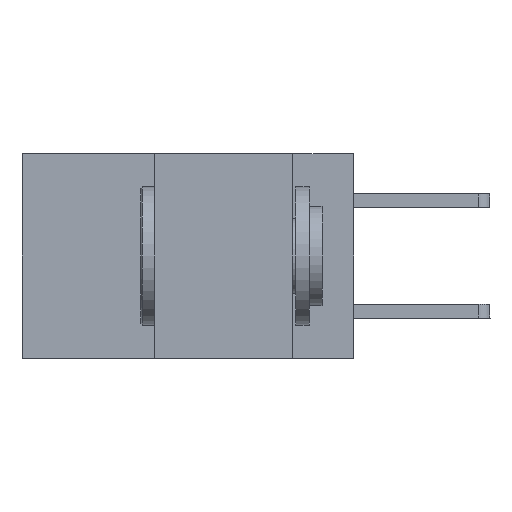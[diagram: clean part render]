
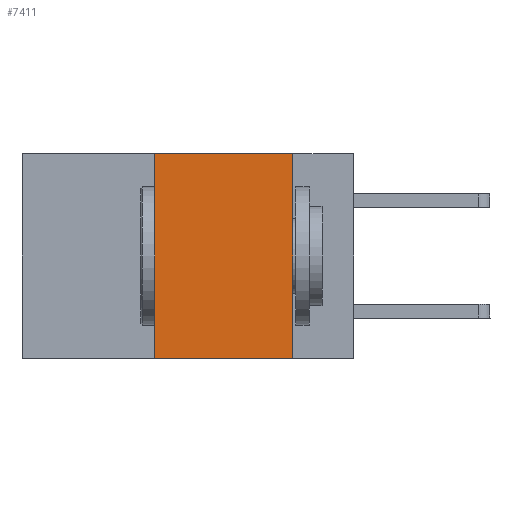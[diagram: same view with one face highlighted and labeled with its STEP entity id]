
A CAD part, left-side view. The second image highlights one B-rep face of the part: STEP entity #7411.
In plain terms, the highlighted planar face has unit normal (-1, 0, 0).
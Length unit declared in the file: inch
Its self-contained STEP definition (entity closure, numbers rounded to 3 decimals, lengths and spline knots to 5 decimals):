
#1052 = DIRECTION ( 'NONE',  ( 0., 0., -1. ) ) ;
#1598 = VERTEX_POINT ( 'NONE', #10853 ) ;
#2135 = AXIS2_PLACEMENT_3D ( 'NONE', #3024, #12877, #7651 ) ;
#2261 = VECTOR ( 'NONE', #1052, 39.37008 ) ;
#2601 = VERTEX_POINT ( 'NONE', #3759 ) ;
#3024 = CARTESIAN_POINT ( 'NONE',  ( 0., 0.6, 0. ) ) ;
#3171 = CARTESIAN_POINT ( 'NONE',  ( 0., 0.36, 0. ) ) ;
#3212 = DIRECTION ( 'NONE',  ( 0., -1., 0. ) ) ;
#3244 = PLANE ( 'NONE',  #2135 ) ;
#3274 = EDGE_CURVE ( 'NONE', #2601, #4172, #4216, .T. ) ;
#3382 = EDGE_CURVE ( 'NONE', #1598, #5369, #4292, .T. ) ;
#3759 = CARTESIAN_POINT ( 'NONE',  ( 0., 0.36, 0. ) ) ;
#3973 = VECTOR ( 'NONE', #10871, 39.37008 ) ;
#4172 = VERTEX_POINT ( 'NONE', #4383 ) ;
#4216 = LINE ( 'NONE', #5590, #7147 ) ;
#4292 = LINE ( 'NONE', #7536, #5637 ) ;
#4383 = CARTESIAN_POINT ( 'NONE',  ( 0., 0.11, 0. ) ) ;
#5017 = EDGE_CURVE ( 'NONE', #4172, #5369, #6732, .T. ) ;
#5369 = VERTEX_POINT ( 'NONE', #9530 ) ;
#5590 = CARTESIAN_POINT ( 'NONE',  ( 0., 0.6, 0. ) ) ;
#5637 = VECTOR ( 'NONE', #3212, 39.37008 ) ;
#5651 = CARTESIAN_POINT ( 'NONE',  ( 0., 0.11, 0. ) ) ;
#6732 = LINE ( 'NONE', #5651, #2261 ) ;
#6970 = ORIENTED_EDGE ( 'NONE', *, *, #3274, .F. ) ;
#7134 = ORIENTED_EDGE ( 'NONE', *, *, #5017, .F. ) ;
#7147 = VECTOR ( 'NONE', #13134, 39.37008 ) ;
#7411 = ADVANCED_FACE ( 'NONE', ( #9583 ), #3244, .F. ) ;
#7536 = CARTESIAN_POINT ( 'NONE',  ( 0., 0.6, -0.37 ) ) ;
#7556 = ORIENTED_EDGE ( 'NONE', *, *, #12556, .F. ) ;
#7651 = DIRECTION ( 'NONE',  ( 0., 0., -1. ) ) ;
#8657 = LINE ( 'NONE', #3171, #3973 ) ;
#9530 = CARTESIAN_POINT ( 'NONE',  ( 0., 0.11, -0.37 ) ) ;
#9579 = ORIENTED_EDGE ( 'NONE', *, *, #3382, .T. ) ;
#9583 = FACE_OUTER_BOUND ( 'NONE', #12719, .T. ) ;
#10853 = CARTESIAN_POINT ( 'NONE',  ( 0., 0.36, -0.37 ) ) ;
#10871 = DIRECTION ( 'NONE',  ( 0., 0., 1. ) ) ;
#12556 = EDGE_CURVE ( 'NONE', #1598, #2601, #8657, .T. ) ;
#12719 = EDGE_LOOP ( 'NONE', ( #7134, #6970, #7556, #9579 ) ) ;
#12877 = DIRECTION ( 'NONE',  ( 1., 0., 0. ) ) ;
#13134 = DIRECTION ( 'NONE',  ( 0., -1., 0. ) ) ;
